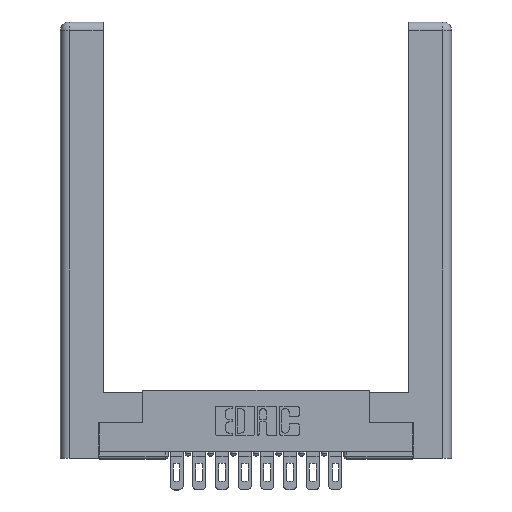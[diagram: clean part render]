
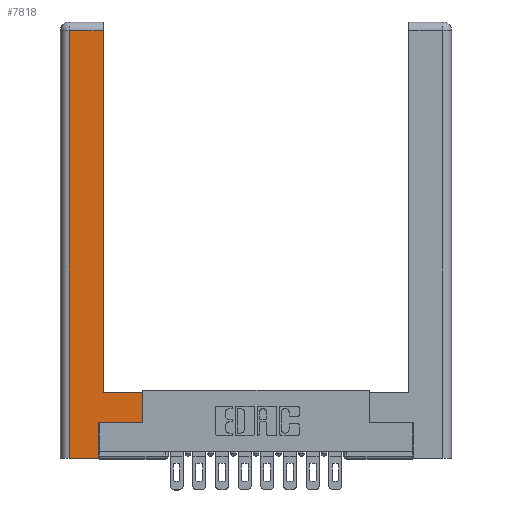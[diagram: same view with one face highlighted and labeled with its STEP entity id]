
A CAD part, top view. The second image highlights one B-rep face of the part: STEP entity #7818.
In plain terms, the highlighted planar face has unit normal (0, 0, 1).
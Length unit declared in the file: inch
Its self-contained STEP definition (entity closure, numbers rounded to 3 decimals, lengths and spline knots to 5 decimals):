
#242 = CARTESIAN_POINT ( 'NONE',  ( 0.265, 0., 0. ) ) ;
#405 = LINE ( 'NONE', #11147, #5296 ) ;
#645 = PLANE ( 'NONE',  #12090 ) ;
#836 = EDGE_CURVE ( 'NONE', #8271, #6175, #7780, .T. ) ;
#942 = FACE_OUTER_BOUND ( 'NONE', #12574, .T. ) ;
#1438 = EDGE_CURVE ( 'NONE', #4531, #8271, #1473, .T. ) ;
#1473 = LINE ( 'NONE', #12372, #11251 ) ;
#1537 = ORIENTED_EDGE ( 'NONE', *, *, #12185, .T. ) ;
#1843 = EDGE_CURVE ( 'NONE', #13755, #12792, #405, .T. ) ;
#1866 = VECTOR ( 'NONE', #11954, 39.37008 ) ;
#1902 = VERTEX_POINT ( 'NONE', #14044 ) ;
#2024 = DIRECTION ( 'NONE',  ( 0., 1., 0. ) ) ;
#2223 = EDGE_CURVE ( 'NONE', #12792, #1902, #13125, .T. ) ;
#2379 = CARTESIAN_POINT ( 'NONE',  ( 0.265, 0.245, 0. ) ) ;
#2899 = ORIENTED_EDGE ( 'NONE', *, *, #1438, .T. ) ;
#3369 = CARTESIAN_POINT ( 'NONE',  ( 0.565, 0.45, 0. ) ) ;
#3650 = LINE ( 'NONE', #11537, #8726 ) ;
#3764 = CARTESIAN_POINT ( 'NONE',  ( 0.295, 0.45, 0. ) ) ;
#3863 = ORIENTED_EDGE ( 'NONE', *, *, #4069, .T. ) ;
#3867 = DIRECTION ( 'NONE',  ( -1., 0., 0. ) ) ;
#4031 = EDGE_CURVE ( 'NONE', #1902, #12752, #3650, .T. ) ;
#4069 = EDGE_CURVE ( 'NONE', #6175, #12450, #11859, .T. ) ;
#4531 = VERTEX_POINT ( 'NONE', #242 ) ;
#4848 = DIRECTION ( 'NONE',  ( 0., 1., 0. ) ) ;
#5296 = VECTOR ( 'NONE', #8020, 39.37008 ) ;
#5577 = VECTOR ( 'NONE', #4848, 39.37008 ) ;
#5681 = VECTOR ( 'NONE', #5993, 39.37008 ) ;
#5993 = DIRECTION ( 'NONE',  ( 1., 0., 0. ) ) ;
#6121 = ORIENTED_EDGE ( 'NONE', *, *, #4031, .T. ) ;
#6175 = VERTEX_POINT ( 'NONE', #14063 ) ;
#6290 = CARTESIAN_POINT ( 'NONE',  ( 0.295, 2.94, 0. ) ) ;
#7780 = LINE ( 'NONE', #13849, #5681 ) ;
#7818 = ADVANCED_FACE ( 'NONE', ( #942 ), #645, .F. ) ;
#7898 = ORIENTED_EDGE ( 'NONE', *, *, #8027, .T. ) ;
#8020 = DIRECTION ( 'NONE',  ( 0., 1., 0. ) ) ;
#8027 = EDGE_CURVE ( 'NONE', #12752, #4531, #13937, .T. ) ;
#8271 = VERTEX_POINT ( 'NONE', #2379 ) ;
#8357 = CARTESIAN_POINT ( 'NONE',  ( 0., 0., 0. ) ) ;
#8726 = VECTOR ( 'NONE', #11588, 39.37008 ) ;
#9016 = ORIENTED_EDGE ( 'NONE', *, *, #836, .T. ) ;
#9619 = DIRECTION ( 'NONE',  ( 0., 0., -1. ) ) ;
#9648 = VECTOR ( 'NONE', #10470, 39.37008 ) ;
#10339 = VECTOR ( 'NONE', #3867, 39.37008 ) ;
#10470 = DIRECTION ( 'NONE',  ( -1., 0., 0. ) ) ;
#10838 = CARTESIAN_POINT ( 'NONE',  ( 0.265, 0., 0. ) ) ;
#11147 = CARTESIAN_POINT ( 'NONE',  ( 0.295, 3., 0. ) ) ;
#11251 = VECTOR ( 'NONE', #2024, 39.37008 ) ;
#11537 = CARTESIAN_POINT ( 'NONE',  ( 0.0615, 0., 0. ) ) ;
#11588 = DIRECTION ( 'NONE',  ( 0., -1., 0. ) ) ;
#11729 = DIRECTION ( 'NONE',  ( -1., 0., 0. ) ) ;
#11859 = LINE ( 'NONE', #13734, #5577 ) ;
#11954 = DIRECTION ( 'NONE',  ( 1., 0., 0. ) ) ;
#12090 = AXIS2_PLACEMENT_3D ( 'NONE', #8357, #9619, #11729 ) ;
#12185 = EDGE_CURVE ( 'NONE', #12450, #13755, #13314, .T. ) ;
#12372 = CARTESIAN_POINT ( 'NONE',  ( 0.265, 0.245, 0. ) ) ;
#12450 = VERTEX_POINT ( 'NONE', #3369 ) ;
#12574 = EDGE_LOOP ( 'NONE', ( #13034, #14277, #6121, #7898, #2899, #9016, #3863, #1537 ) ) ;
#12730 = CARTESIAN_POINT ( 'NONE',  ( 0.0615, 0., 0. ) ) ;
#12752 = VERTEX_POINT ( 'NONE', #12730 ) ;
#12792 = VERTEX_POINT ( 'NONE', #6290 ) ;
#13034 = ORIENTED_EDGE ( 'NONE', *, *, #1843, .T. ) ;
#13125 = LINE ( 'NONE', #13984, #9648 ) ;
#13251 = CARTESIAN_POINT ( 'NONE',  ( 0.295, 0.45, 0. ) ) ;
#13314 = LINE ( 'NONE', #3764, #10339 ) ;
#13734 = CARTESIAN_POINT ( 'NONE',  ( 0.565, 0.45, 0. ) ) ;
#13755 = VERTEX_POINT ( 'NONE', #13251 ) ;
#13849 = CARTESIAN_POINT ( 'NONE',  ( 0.565, 0.245, 0. ) ) ;
#13937 = LINE ( 'NONE', #10838, #1866 ) ;
#13984 = CARTESIAN_POINT ( 'NONE',  ( 0.0615, 2.94, 0. ) ) ;
#14044 = CARTESIAN_POINT ( 'NONE',  ( 0.0615, 2.94, 0. ) ) ;
#14063 = CARTESIAN_POINT ( 'NONE',  ( 0.565, 0.245, 0. ) ) ;
#14277 = ORIENTED_EDGE ( 'NONE', *, *, #2223, .T. ) ;
